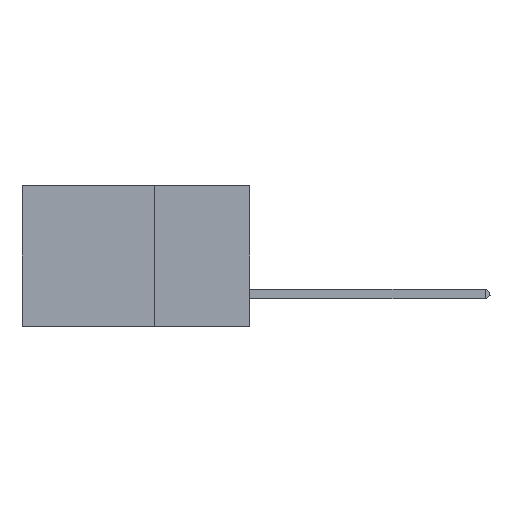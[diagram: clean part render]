
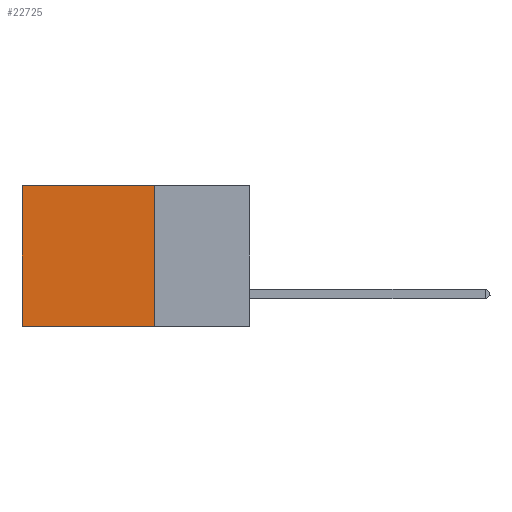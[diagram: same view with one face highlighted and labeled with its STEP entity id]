
A CAD part, left-side view. The second image highlights one B-rep face of the part: STEP entity #22725.
In plain terms, the highlighted planar face has unit normal (-1, 0, 0).
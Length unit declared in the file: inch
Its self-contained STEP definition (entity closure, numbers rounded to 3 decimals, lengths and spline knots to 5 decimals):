
#134 = FACE_OUTER_BOUND ( 'NONE', #3083, .T. ) ;
#276 = ORIENTED_EDGE ( 'NONE', *, *, #14091, .F. ) ;
#1271 = CARTESIAN_POINT ( 'NONE',  ( 0.2875, 0.25, -0.37 ) ) ;
#1982 = CARTESIAN_POINT ( 'NONE',  ( 0.2875, 0.25, 0. ) ) ;
#3083 = EDGE_LOOP ( 'NONE', ( #20267, #276, #7015, #17936 ) ) ;
#4589 = DIRECTION ( 'NONE',  ( 0., 1., 0. ) ) ;
#6189 = DIRECTION ( 'NONE',  ( 0., 0., -1. ) ) ;
#7015 = ORIENTED_EDGE ( 'NONE', *, *, #8359, .F. ) ;
#7030 = VECTOR ( 'NONE', #4589, 39.37008 ) ;
#7052 = AXIS2_PLACEMENT_3D ( 'NONE', #1982, #30107, #25239 ) ;
#8359 = EDGE_CURVE ( 'NONE', #13746, #22039, #32055, .T. ) ;
#9844 = LINE ( 'NONE', #18915, #23331 ) ;
#11071 = CARTESIAN_POINT ( 'NONE',  ( 0.2875, 0.6, 0. ) ) ;
#13746 = VERTEX_POINT ( 'NONE', #25207 ) ;
#14051 = EDGE_CURVE ( 'NONE', #13746, #19496, #28768, .T. ) ;
#14091 = EDGE_CURVE ( 'NONE', #22039, #26241, #32774, .T. ) ;
#14845 = CARTESIAN_POINT ( 'NONE',  ( 0.2875, 0.25, 0. ) ) ;
#17137 = CARTESIAN_POINT ( 'NONE',  ( 0.2875, 0.25, 0. ) ) ;
#17936 = ORIENTED_EDGE ( 'NONE', *, *, #14051, .T. ) ;
#18915 = CARTESIAN_POINT ( 'NONE',  ( 0.2875, 0.6, 0. ) ) ;
#19496 = VERTEX_POINT ( 'NONE', #11071 ) ;
#19643 = EDGE_CURVE ( 'NONE', #19496, #26241, #9844, .T. ) ;
#20267 = ORIENTED_EDGE ( 'NONE', *, *, #19643, .T. ) ;
#22039 = VERTEX_POINT ( 'NONE', #22796 ) ;
#22271 = PLANE ( 'NONE',  #7052 ) ;
#22725 = ADVANCED_FACE ( 'NONE', ( #134 ), #22271, .F. ) ;
#22796 = CARTESIAN_POINT ( 'NONE',  ( 0.2875, 0.25, -0.37 ) ) ;
#23331 = VECTOR ( 'NONE', #6189, 39.37008 ) ;
#25207 = CARTESIAN_POINT ( 'NONE',  ( 0.2875, 0.25, 0. ) ) ;
#25239 = DIRECTION ( 'NONE',  ( 0., 0., -1. ) ) ;
#26241 = VERTEX_POINT ( 'NONE', #30687 ) ;
#26727 = DIRECTION ( 'NONE',  ( 0., 1., 0. ) ) ;
#27618 = VECTOR ( 'NONE', #26727, 39.37008 ) ;
#28768 = LINE ( 'NONE', #17137, #7030 ) ;
#29659 = VECTOR ( 'NONE', #30320, 39.37008 ) ;
#30107 = DIRECTION ( 'NONE',  ( 1., 0., 0. ) ) ;
#30320 = DIRECTION ( 'NONE',  ( 0., 0., -1. ) ) ;
#30687 = CARTESIAN_POINT ( 'NONE',  ( 0.2875, 0.6, -0.37 ) ) ;
#32055 = LINE ( 'NONE', #14845, #29659 ) ;
#32774 = LINE ( 'NONE', #1271, #27618 ) ;
